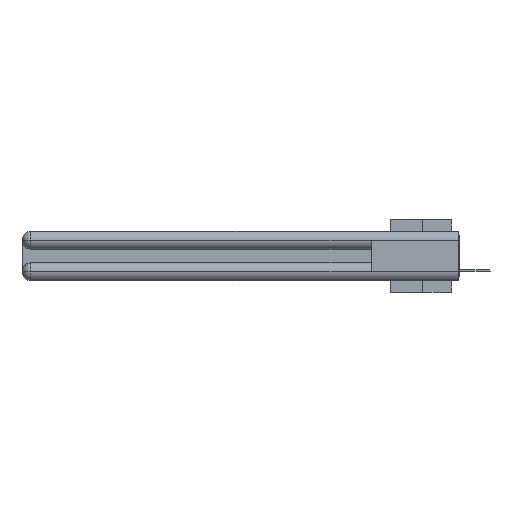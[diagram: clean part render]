
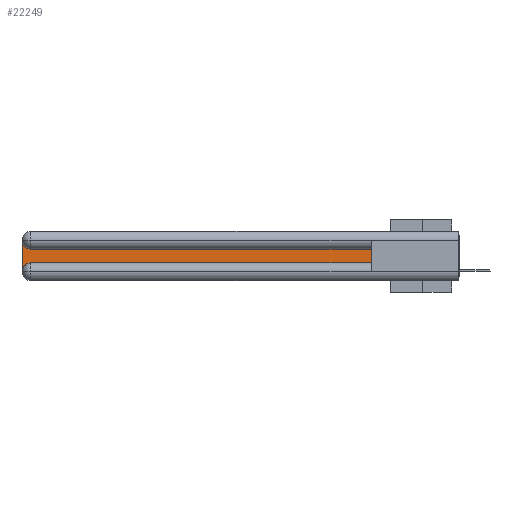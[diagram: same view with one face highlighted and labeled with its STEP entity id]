
A CAD part, left-side view. The second image highlights one B-rep face of the part: STEP entity #22249.
In plain terms, the highlighted planar face has unit normal (-1, 0, 0).
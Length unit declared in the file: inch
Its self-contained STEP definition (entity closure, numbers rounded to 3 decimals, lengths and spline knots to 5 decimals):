
#1835 = VECTOR ( 'NONE', #23618, 39.37008 ) ;
#2237 = DIRECTION ( 'NONE',  ( 0., 0., -1. ) ) ;
#2538 = CARTESIAN_POINT ( 'NONE',  ( 0.075, 2.94, -0.2775 ) ) ;
#3448 = VECTOR ( 'NONE', #16930, 39.37008 ) ;
#3924 = CARTESIAN_POINT ( 'NONE',  ( 0.075, 0.6, -0.1225 ) ) ;
#4394 = ORIENTED_EDGE ( 'NONE', *, *, #19235, .T. ) ;
#5360 = CARTESIAN_POINT ( 'NONE',  ( 0.075, 3., -0.0625 ) ) ;
#5513 = CARTESIAN_POINT ( 'NONE',  ( 0.075, 0.6, -0.1225 ) ) ;
#6710 = CARTESIAN_POINT ( 'NONE',  ( 0.075, 2.94, -0.1225 ) ) ;
#7558 = CARTESIAN_POINT ( 'NONE',  ( 0.075, 2.94, -0.2175 ) ) ;
#8149 = DIRECTION ( 'NONE',  ( 0., 0., -1. ) ) ;
#8791 = LINE ( 'NONE', #3924, #1835 ) ;
#9059 = CARTESIAN_POINT ( 'NONE',  ( 0.075, 2.94, -0.0625 ) ) ;
#10145 = AXIS2_PLACEMENT_3D ( 'NONE', #9059, #19263, #17100 ) ;
#12763 = VERTEX_POINT ( 'NONE', #5513 ) ;
#13732 = CARTESIAN_POINT ( 'NONE',  ( 0.075, 0.6, -0.2175 ) ) ;
#14287 = AXIS2_PLACEMENT_3D ( 'NONE', #2538, #22443, #8149 ) ;
#15704 = LINE ( 'NONE', #13732, #22763 ) ;
#15706 = EDGE_LOOP ( 'NONE', ( #23350, #29458, #36055, #28911, #32535, #4394 ) ) ;
#16885 = EDGE_CURVE ( 'NONE', #23996, #32266, #31202, .T. ) ;
#16930 = DIRECTION ( 'NONE',  ( 0., 0., -1. ) ) ;
#17100 = DIRECTION ( 'NONE',  ( 0., 0., -1. ) ) ;
#18117 = AXIS2_PLACEMENT_3D ( 'NONE', #33078, #35873, #2237 ) ;
#18120 = FACE_OUTER_BOUND ( 'NONE', #15706, .T. ) ;
#19060 = CARTESIAN_POINT ( 'NONE',  ( 0.075, 3., -0.2775 ) ) ;
#19235 = EDGE_CURVE ( 'NONE', #19870, #12763, #15704, .T. ) ;
#19263 = DIRECTION ( 'NONE',  ( 1., 0., 0. ) ) ;
#19323 = PLANE ( 'NONE',  #18117 ) ;
#19591 = CIRCLE ( 'NONE', #10145, 0.06 ) ;
#19870 = VERTEX_POINT ( 'NONE', #22752 ) ;
#22249 = ADVANCED_FACE ( 'NONE', ( #18120 ), #19323, .F. ) ;
#22443 = DIRECTION ( 'NONE',  ( 1., 0., 0. ) ) ;
#22752 = CARTESIAN_POINT ( 'NONE',  ( 0.075, 0.6, -0.2175 ) ) ;
#22763 = VECTOR ( 'NONE', #33137, 39.37008 ) ;
#22908 = CIRCLE ( 'NONE', #14287, 0.06 ) ;
#22960 = EDGE_CURVE ( 'NONE', #12763, #27002, #8791, .T. ) ;
#23350 = ORIENTED_EDGE ( 'NONE', *, *, #22960, .T. ) ;
#23618 = DIRECTION ( 'NONE',  ( 0., 1., 0. ) ) ;
#23996 = VERTEX_POINT ( 'NONE', #5360 ) ;
#27002 = VERTEX_POINT ( 'NONE', #6710 ) ;
#27092 = VERTEX_POINT ( 'NONE', #7558 ) ;
#27878 = EDGE_CURVE ( 'NONE', #27092, #19870, #27933, .T. ) ;
#27933 = LINE ( 'NONE', #30182, #30970 ) ;
#28282 = CARTESIAN_POINT ( 'NONE',  ( 0.075, 3., -0.2175 ) ) ;
#28911 = ORIENTED_EDGE ( 'NONE', *, *, #30348, .T. ) ;
#29458 = ORIENTED_EDGE ( 'NONE', *, *, #36231, .T. ) ;
#30182 = CARTESIAN_POINT ( 'NONE',  ( 0.075, 0.6, -0.2175 ) ) ;
#30348 = EDGE_CURVE ( 'NONE', #32266, #27092, #22908, .T. ) ;
#30970 = VECTOR ( 'NONE', #32882, 39.37008 ) ;
#31202 = LINE ( 'NONE', #28282, #3448 ) ;
#32266 = VERTEX_POINT ( 'NONE', #19060 ) ;
#32535 = ORIENTED_EDGE ( 'NONE', *, *, #27878, .T. ) ;
#32882 = DIRECTION ( 'NONE',  ( 0., -1., 0. ) ) ;
#33078 = CARTESIAN_POINT ( 'NONE',  ( 0.075, 3., -0.1225 ) ) ;
#33137 = DIRECTION ( 'NONE',  ( 0., 0., 1. ) ) ;
#35873 = DIRECTION ( 'NONE',  ( 1., 0., 0. ) ) ;
#36055 = ORIENTED_EDGE ( 'NONE', *, *, #16885, .T. ) ;
#36231 = EDGE_CURVE ( 'NONE', #27002, #23996, #19591, .T. ) ;
